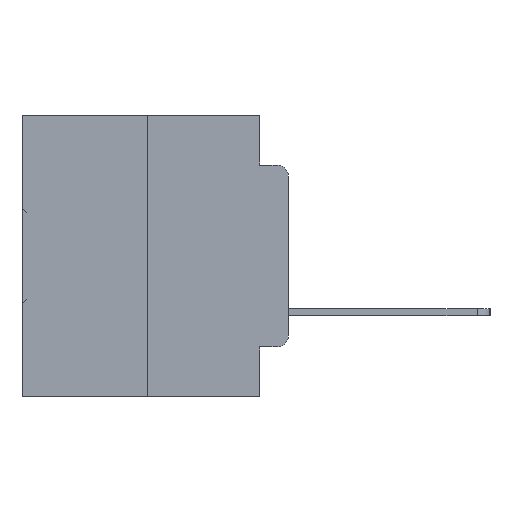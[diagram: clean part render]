
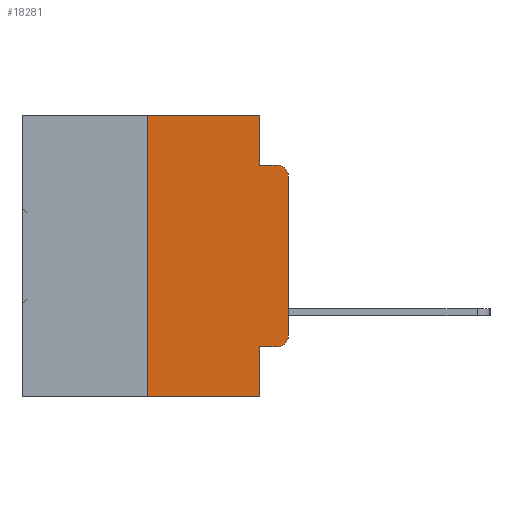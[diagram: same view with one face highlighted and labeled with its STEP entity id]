
A CAD part, left-side view. The second image highlights one B-rep face of the part: STEP entity #18281.
In plain terms, the highlighted planar face has unit normal (-1, 0, 0).
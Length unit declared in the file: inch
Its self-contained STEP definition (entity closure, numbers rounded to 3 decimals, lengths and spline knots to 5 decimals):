
#887 = FACE_OUTER_BOUND ( 'NONE', #26121, .T. ) ;
#1067 = CARTESIAN_POINT ( 'NONE',  ( 0., 0.02, -0.0885 ) ) ;
#1234 = VERTEX_POINT ( 'NONE', #29498 ) ;
#1317 = ORIENTED_EDGE ( 'NONE', *, *, #6941, .T. ) ;
#1505 = CIRCLE ( 'NONE', #20048, 0.02 ) ;
#1539 = EDGE_CURVE ( 'NONE', #13603, #6971, #3067, .T. ) ;
#1545 = VERTEX_POINT ( 'NONE', #9639 ) ;
#1759 = ORIENTED_EDGE ( 'NONE', *, *, #11184, .T. ) ;
#1791 = DIRECTION ( 'NONE',  ( 0., 0., -1. ) ) ;
#2005 = CARTESIAN_POINT ( 'NONE',  ( 0., 0.473, 0. ) ) ;
#3061 = VERTEX_POINT ( 'NONE', #28543 ) ;
#3067 = LINE ( 'NONE', #22694, #29541 ) ;
#3525 = LINE ( 'NONE', #9645, #23084 ) ;
#3617 = DIRECTION ( 'NONE',  ( 0., -1., 0. ) ) ;
#3965 = LINE ( 'NONE', #20148, #31203 ) ;
#4267 = DIRECTION ( 'NONE',  ( 0., 0., 1. ) ) ;
#4684 = ORIENTED_EDGE ( 'NONE', *, *, #11278, .F. ) ;
#6148 = LINE ( 'NONE', #7577, #20301 ) ;
#6735 = CARTESIAN_POINT ( 'NONE',  ( 0., 0.25, -0.5 ) ) ;
#6933 = DIRECTION ( 'NONE',  ( 0., -1., 0. ) ) ;
#6941 = EDGE_CURVE ( 'NONE', #3061, #20583, #8266, .T. ) ;
#6971 = VERTEX_POINT ( 'NONE', #21794 ) ;
#7170 = DIRECTION ( 'NONE',  ( 0., -1., 0. ) ) ;
#7263 = ORIENTED_EDGE ( 'NONE', *, *, #28091, .F. ) ;
#7351 = AXIS2_PLACEMENT_3D ( 'NONE', #2005, #25982, #10184 ) ;
#7577 = CARTESIAN_POINT ( 'NONE',  ( 0., 0.473, 0. ) ) ;
#8239 = EDGE_CURVE ( 'NONE', #24747, #1545, #27550, .T. ) ;
#8266 = CIRCLE ( 'NONE', #25241, 0.02 ) ;
#8932 = CARTESIAN_POINT ( 'NONE',  ( 0., 0.051, -0.0885 ) ) ;
#9611 = CARTESIAN_POINT ( 'NONE',  ( 0., 0., 0. ) ) ;
#9639 = CARTESIAN_POINT ( 'NONE',  ( 0., 0.02, -0.4115 ) ) ;
#9645 = CARTESIAN_POINT ( 'NONE',  ( 0., 0.473, -0.5 ) ) ;
#10184 = DIRECTION ( 'NONE',  ( 0., 0., -1. ) ) ;
#11184 = EDGE_CURVE ( 'NONE', #1545, #23579, #1505, .T. ) ;
#11192 = CARTESIAN_POINT ( 'NONE',  ( 0., 0.02, -0.1085 ) ) ;
#11278 = EDGE_CURVE ( 'NONE', #6971, #30595, #6148, .T. ) ;
#12859 = VECTOR ( 'NONE', #4267, 39.37008 ) ;
#13120 = VERTEX_POINT ( 'NONE', #25646 ) ;
#13603 = VERTEX_POINT ( 'NONE', #6735 ) ;
#13837 = DIRECTION ( 'NONE',  ( 0., 0., -1. ) ) ;
#14097 = DIRECTION ( 'NONE',  ( 0., 0., -1. ) ) ;
#14240 = EDGE_CURVE ( 'NONE', #13603, #13120, #3525, .T. ) ;
#14413 = VECTOR ( 'NONE', #7170, 39.37008 ) ;
#15533 = EDGE_CURVE ( 'NONE', #1234, #20583, #18808, .T. ) ;
#16415 = ORIENTED_EDGE ( 'NONE', *, *, #15533, .F. ) ;
#16766 = CARTESIAN_POINT ( 'NONE',  ( 0., 0.051, 0. ) ) ;
#17129 = VECTOR ( 'NONE', #14097, 39.37008 ) ;
#17834 = DIRECTION ( 'NONE',  ( -1., 0., 0. ) ) ;
#18281 = ADVANCED_FACE ( 'NONE', ( #887 ), #23323, .F. ) ;
#18808 = LINE ( 'NONE', #8932, #32638 ) ;
#18884 = ORIENTED_EDGE ( 'NONE', *, *, #1539, .F. ) ;
#19897 = LINE ( 'NONE', #9611, #12859 ) ;
#20048 = AXIS2_PLACEMENT_3D ( 'NONE', #33372, #17834, #1791 ) ;
#20148 = CARTESIAN_POINT ( 'NONE',  ( 0., 0.051, 0. ) ) ;
#20301 = VECTOR ( 'NONE', #33829, 39.37008 ) ;
#20540 = ORIENTED_EDGE ( 'NONE', *, *, #14240, .T. ) ;
#20583 = VERTEX_POINT ( 'NONE', #1067 ) ;
#21794 = CARTESIAN_POINT ( 'NONE',  ( 0., 0.25, 0. ) ) ;
#22694 = CARTESIAN_POINT ( 'NONE',  ( 0., 0.25, 0. ) ) ;
#22784 = DIRECTION ( 'NONE',  ( 0., 0., -1. ) ) ;
#23048 = CARTESIAN_POINT ( 'NONE',  ( 0., 0.051, -0.4115 ) ) ;
#23084 = VECTOR ( 'NONE', #6933, 39.37008 ) ;
#23323 = PLANE ( 'NONE',  #7351 ) ;
#23579 = VERTEX_POINT ( 'NONE', #29819 ) ;
#24110 = LINE ( 'NONE', #16766, #17129 ) ;
#24747 = VERTEX_POINT ( 'NONE', #31997 ) ;
#25241 = AXIS2_PLACEMENT_3D ( 'NONE', #11192, #29530, #13837 ) ;
#25646 = CARTESIAN_POINT ( 'NONE',  ( 0., 0.051, -0.5 ) ) ;
#25982 = DIRECTION ( 'NONE',  ( 1., 0., 0. ) ) ;
#26004 = CARTESIAN_POINT ( 'NONE',  ( 0., 0.051, 0. ) ) ;
#26121 = EDGE_LOOP ( 'NONE', ( #33097, #1317, #16415, #30321, #4684, #18884, #20540, #7263, #29101, #1759 ) ) ;
#27550 = LINE ( 'NONE', #23048, #14413 ) ;
#28091 = EDGE_CURVE ( 'NONE', #24747, #13120, #3965, .T. ) ;
#28543 = CARTESIAN_POINT ( 'NONE',  ( 0., 0., -0.1085 ) ) ;
#29101 = ORIENTED_EDGE ( 'NONE', *, *, #8239, .T. ) ;
#29498 = CARTESIAN_POINT ( 'NONE',  ( 0., 0.051, -0.0885 ) ) ;
#29530 = DIRECTION ( 'NONE',  ( -1., 0., 0. ) ) ;
#29541 = VECTOR ( 'NONE', #33077, 39.37008 ) ;
#29819 = CARTESIAN_POINT ( 'NONE',  ( 0., 0., -0.3915 ) ) ;
#30321 = ORIENTED_EDGE ( 'NONE', *, *, #31672, .F. ) ;
#30595 = VERTEX_POINT ( 'NONE', #26004 ) ;
#31203 = VECTOR ( 'NONE', #22784, 39.37008 ) ;
#31672 = EDGE_CURVE ( 'NONE', #30595, #1234, #24110, .T. ) ;
#31997 = CARTESIAN_POINT ( 'NONE',  ( 0., 0.051, -0.4115 ) ) ;
#32638 = VECTOR ( 'NONE', #3617, 39.37008 ) ;
#33026 = EDGE_CURVE ( 'NONE', #23579, #3061, #19897, .T. ) ;
#33077 = DIRECTION ( 'NONE',  ( 0., 0., 1. ) ) ;
#33097 = ORIENTED_EDGE ( 'NONE', *, *, #33026, .T. ) ;
#33372 = CARTESIAN_POINT ( 'NONE',  ( 0., 0.02, -0.3915 ) ) ;
#33829 = DIRECTION ( 'NONE',  ( 0., -1., 0. ) ) ;
